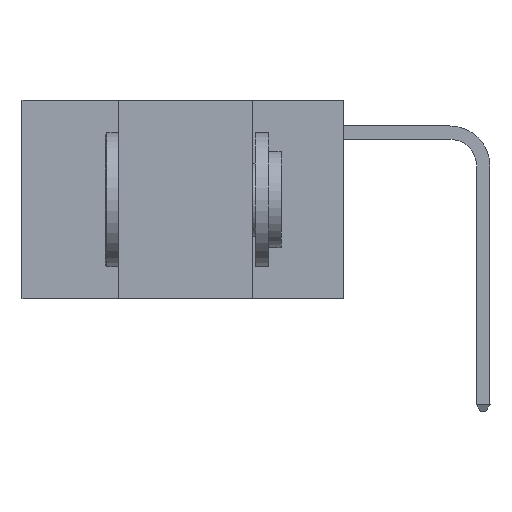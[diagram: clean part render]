
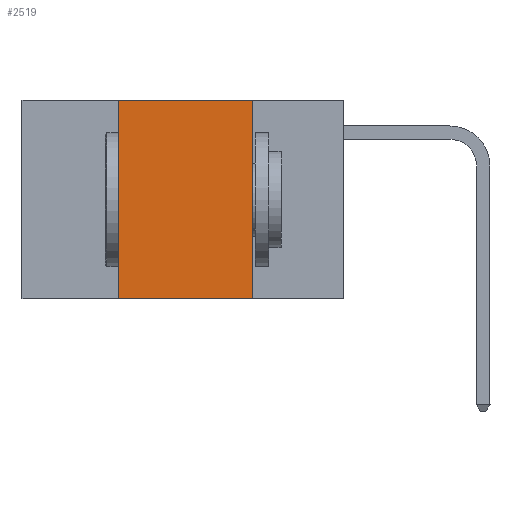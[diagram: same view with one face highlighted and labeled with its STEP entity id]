
A CAD part, left-side view. The second image highlights one B-rep face of the part: STEP entity #2519.
In plain terms, the highlighted planar face has unit normal (-1, 0, 0).
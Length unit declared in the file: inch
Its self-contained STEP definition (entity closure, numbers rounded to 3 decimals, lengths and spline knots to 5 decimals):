
#47 = CARTESIAN_POINT ( 'NONE',  ( 0., 0.17, 0. ) ) ;
#99 = CARTESIAN_POINT ( 'NONE',  ( 0., 0.6, 0. ) ) ;
#382 = AXIS2_PLACEMENT_3D ( 'NONE', #99, #4345, #11818 ) ;
#407 = CARTESIAN_POINT ( 'NONE',  ( 0., 0.17, -0.37 ) ) ;
#1200 = PLANE ( 'NONE',  #382 ) ;
#1222 = DIRECTION ( 'NONE',  ( 0., 0., 1. ) ) ;
#1339 = LINE ( 'NONE', #9793, #11569 ) ;
#2219 = VERTEX_POINT ( 'NONE', #8863 ) ;
#2519 = ADVANCED_FACE ( 'NONE', ( #7599 ), #1200, .F. ) ;
#3459 = LINE ( 'NONE', #7689, #3779 ) ;
#3779 = VECTOR ( 'NONE', #1222, 39.37008 ) ;
#3788 = LINE ( 'NONE', #5979, #11728 ) ;
#4165 = CARTESIAN_POINT ( 'NONE',  ( 0., 0.6, 0. ) ) ;
#4260 = EDGE_CURVE ( 'NONE', #8335, #12068, #3788, .T. ) ;
#4345 = DIRECTION ( 'NONE',  ( 1., 0., 0. ) ) ;
#4357 = CARTESIAN_POINT ( 'NONE',  ( 0., 0.42, -0.37 ) ) ;
#5979 = CARTESIAN_POINT ( 'NONE',  ( 0., 0.17, 0. ) ) ;
#7068 = EDGE_LOOP ( 'NONE', ( #8314, #8698, #13489, #11225 ) ) ;
#7401 = DIRECTION ( 'NONE',  ( 0., -1., 0. ) ) ;
#7599 = FACE_OUTER_BOUND ( 'NONE', #7068, .T. ) ;
#7689 = CARTESIAN_POINT ( 'NONE',  ( 0., 0.42, 0. ) ) ;
#7800 = DIRECTION ( 'NONE',  ( 0., -1., 0. ) ) ;
#8314 = ORIENTED_EDGE ( 'NONE', *, *, #4260, .F. ) ;
#8335 = VERTEX_POINT ( 'NONE', #47 ) ;
#8360 = EDGE_CURVE ( 'NONE', #2219, #8335, #10381, .T. ) ;
#8698 = ORIENTED_EDGE ( 'NONE', *, *, #8360, .F. ) ;
#8863 = CARTESIAN_POINT ( 'NONE',  ( 0., 0.42, 0. ) ) ;
#9697 = EDGE_CURVE ( 'NONE', #13599, #2219, #3459, .T. ) ;
#9793 = CARTESIAN_POINT ( 'NONE',  ( 0., 0.6, -0.37 ) ) ;
#10013 = DIRECTION ( 'NONE',  ( 0., 0., -1. ) ) ;
#10381 = LINE ( 'NONE', #4165, #12623 ) ;
#11040 = EDGE_CURVE ( 'NONE', #13599, #12068, #1339, .T. ) ;
#11225 = ORIENTED_EDGE ( 'NONE', *, *, #11040, .T. ) ;
#11569 = VECTOR ( 'NONE', #7800, 39.37008 ) ;
#11728 = VECTOR ( 'NONE', #10013, 39.37008 ) ;
#11818 = DIRECTION ( 'NONE',  ( 0., 0., -1. ) ) ;
#12068 = VERTEX_POINT ( 'NONE', #407 ) ;
#12623 = VECTOR ( 'NONE', #7401, 39.37008 ) ;
#13489 = ORIENTED_EDGE ( 'NONE', *, *, #9697, .F. ) ;
#13599 = VERTEX_POINT ( 'NONE', #4357 ) ;
